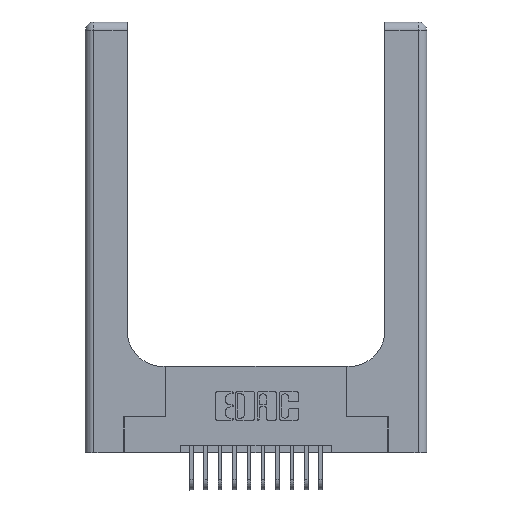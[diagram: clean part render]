
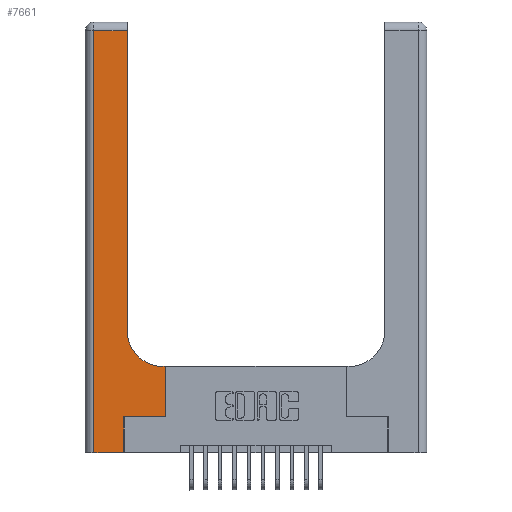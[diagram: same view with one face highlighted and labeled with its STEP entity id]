
A CAD part, top view. The second image highlights one B-rep face of the part: STEP entity #7661.
In plain terms, the highlighted planar face has unit normal (0, 0, 1).
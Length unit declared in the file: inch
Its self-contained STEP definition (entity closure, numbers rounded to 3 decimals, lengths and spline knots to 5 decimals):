
#56 = EDGE_CURVE ( 'NONE', #5082, #8676, #5612, .T. ) ;
#114 = VERTEX_POINT ( 'NONE', #5175 ) ;
#455 = CIRCLE ( 'NONE', #6109, 0.25 ) ;
#584 = CARTESIAN_POINT ( 'NONE',  ( 0.2915, 3., 0.37 ) ) ;
#844 = VECTOR ( 'NONE', #15844, 39.37008 ) ;
#980 = EDGE_CURVE ( 'NONE', #114, #7353, #455, .T. ) ;
#1261 = ORIENTED_EDGE ( 'NONE', *, *, #6124, .T. ) ;
#1282 = DIRECTION ( 'NONE',  ( 0., 0., -1. ) ) ;
#1496 = CARTESIAN_POINT ( 'NONE',  ( 0.269, 0.25, 0.37 ) ) ;
#1539 = VECTOR ( 'NONE', #5350, 39.37008 ) ;
#2049 = ORIENTED_EDGE ( 'NONE', *, *, #56, .T. ) ;
#2068 = DIRECTION ( 'NONE',  ( 0., 1., 0. ) ) ;
#3288 = EDGE_CURVE ( 'NONE', #11733, #114, #4505, .T. ) ;
#3289 = EDGE_CURVE ( 'NONE', #8676, #6404, #9232, .T. ) ;
#3300 = FACE_OUTER_BOUND ( 'NONE', #12291, .T. ) ;
#3795 = EDGE_CURVE ( 'NONE', #5875, #15221, #14474, .T. ) ;
#4166 = CARTESIAN_POINT ( 'NONE',  ( 0.06, 3., 0.37 ) ) ;
#4505 = LINE ( 'NONE', #8097, #844 ) ;
#4778 = CARTESIAN_POINT ( 'NONE',  ( 0.2915, 0.85, 0.37 ) ) ;
#5082 = VERTEX_POINT ( 'NONE', #9017 ) ;
#5175 = CARTESIAN_POINT ( 'NONE',  ( 0.5415, 0.6, 0.37 ) ) ;
#5350 = DIRECTION ( 'NONE',  ( -1., 0., 0. ) ) ;
#5395 = ORIENTED_EDGE ( 'NONE', *, *, #7808, .T. ) ;
#5612 = LINE ( 'NONE', #9088, #1539 ) ;
#5621 = DIRECTION ( 'NONE',  ( 1., 0., 0. ) ) ;
#5875 = VERTEX_POINT ( 'NONE', #10663 ) ;
#5887 = VECTOR ( 'NONE', #2068, 39.37008 ) ;
#5973 = AXIS2_PLACEMENT_3D ( 'NONE', #14449, #1282, #10598 ) ;
#6082 = EDGE_CURVE ( 'NONE', #7353, #5082, #16217, .T. ) ;
#6085 = VECTOR ( 'NONE', #15566, 39.37008 ) ;
#6109 = AXIS2_PLACEMENT_3D ( 'NONE', #13568, #12996, #12827 ) ;
#6124 = EDGE_CURVE ( 'NONE', #15221, #11733, #11976, .T. ) ;
#6404 = VERTEX_POINT ( 'NONE', #16001 ) ;
#6941 = DIRECTION ( 'NONE',  ( 0., 1., 0. ) ) ;
#7353 = VERTEX_POINT ( 'NONE', #4778 ) ;
#7661 = ADVANCED_FACE ( 'NONE', ( #3300 ), #10539, .F. ) ;
#7808 = EDGE_CURVE ( 'NONE', #14358, #5875, #11719, .T. ) ;
#7810 = ORIENTED_EDGE ( 'NONE', *, *, #980, .T. ) ;
#7872 = CARTESIAN_POINT ( 'NONE',  ( 0., 0., 0.37 ) ) ;
#8006 = VECTOR ( 'NONE', #14607, 39.37008 ) ;
#8097 = CARTESIAN_POINT ( 'NONE',  ( 0.2915, 0.6, 0.37 ) ) ;
#8165 = ORIENTED_EDGE ( 'NONE', *, *, #3795, .T. ) ;
#8676 = VERTEX_POINT ( 'NONE', #15254 ) ;
#9017 = CARTESIAN_POINT ( 'NONE',  ( 0.2915, 2.94, 0.37 ) ) ;
#9088 = CARTESIAN_POINT ( 'NONE',  ( 0., 2.94, 0.37 ) ) ;
#9232 = LINE ( 'NONE', #4166, #8006 ) ;
#9325 = ORIENTED_EDGE ( 'NONE', *, *, #3288, .T. ) ;
#9564 = LINE ( 'NONE', #7872, #6085 ) ;
#9772 = ORIENTED_EDGE ( 'NONE', *, *, #15754, .T. ) ;
#9922 = DIRECTION ( 'NONE',  ( 0., 1., 0. ) ) ;
#10539 = PLANE ( 'NONE',  #5973 ) ;
#10598 = DIRECTION ( 'NONE',  ( -1., 0., 0. ) ) ;
#10609 = CARTESIAN_POINT ( 'NONE',  ( 0.5585, 0.25, 0.37 ) ) ;
#10663 = CARTESIAN_POINT ( 'NONE',  ( 0.269, 0.25, 0.37 ) ) ;
#10810 = CARTESIAN_POINT ( 'NONE',  ( 0.269, 0., 0.37 ) ) ;
#11321 = CARTESIAN_POINT ( 'NONE',  ( 0.5585, 0.25, 0.37 ) ) ;
#11719 = LINE ( 'NONE', #10810, #14756 ) ;
#11733 = VERTEX_POINT ( 'NONE', #15747 ) ;
#11976 = LINE ( 'NONE', #11321, #5887 ) ;
#12291 = EDGE_LOOP ( 'NONE', ( #15250, #2049, #13407, #9772, #5395, #8165, #1261, #9325, #7810 ) ) ;
#12827 = DIRECTION ( 'NONE',  ( 1., 0., 0. ) ) ;
#12996 = DIRECTION ( 'NONE',  ( 0., 0., -1. ) ) ;
#13407 = ORIENTED_EDGE ( 'NONE', *, *, #3289, .T. ) ;
#13568 = CARTESIAN_POINT ( 'NONE',  ( 0.5415, 0.85, 0.37 ) ) ;
#13689 = VECTOR ( 'NONE', #5621, 39.37008 ) ;
#14358 = VERTEX_POINT ( 'NONE', #16038 ) ;
#14449 = CARTESIAN_POINT ( 'NONE',  ( 0., 3., 0.37 ) ) ;
#14474 = LINE ( 'NONE', #1496, #13689 ) ;
#14607 = DIRECTION ( 'NONE',  ( 0., -1., 0. ) ) ;
#14756 = VECTOR ( 'NONE', #6941, 39.37008 ) ;
#15221 = VERTEX_POINT ( 'NONE', #10609 ) ;
#15250 = ORIENTED_EDGE ( 'NONE', *, *, #6082, .T. ) ;
#15254 = CARTESIAN_POINT ( 'NONE',  ( 0.06, 2.94, 0.37 ) ) ;
#15566 = DIRECTION ( 'NONE',  ( 1., 0., 0. ) ) ;
#15747 = CARTESIAN_POINT ( 'NONE',  ( 0.5585, 0.6, 0.37 ) ) ;
#15754 = EDGE_CURVE ( 'NONE', #6404, #14358, #9564, .T. ) ;
#15844 = DIRECTION ( 'NONE',  ( -1., 0., 0. ) ) ;
#16001 = CARTESIAN_POINT ( 'NONE',  ( 0.06, 0., 0.37 ) ) ;
#16038 = CARTESIAN_POINT ( 'NONE',  ( 0.269, 0., 0.37 ) ) ;
#16217 = LINE ( 'NONE', #584, #16629 ) ;
#16629 = VECTOR ( 'NONE', #9922, 39.37008 ) ;
